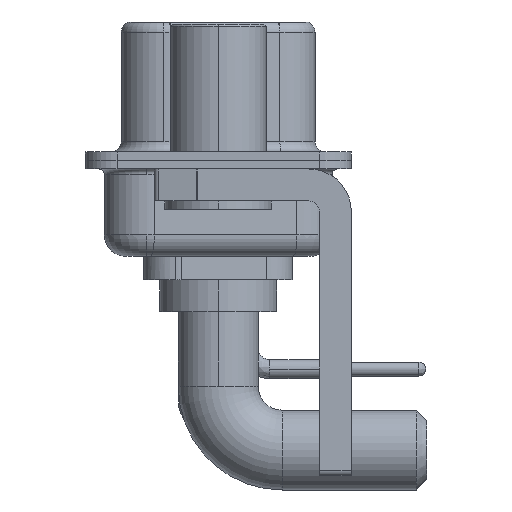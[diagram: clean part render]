
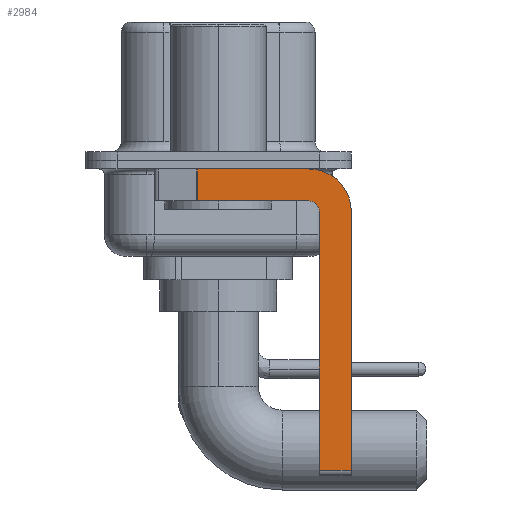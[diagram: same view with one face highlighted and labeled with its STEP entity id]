
A CAD part, left-side view. The second image highlights one B-rep face of the part: STEP entity #2984.
In plain terms, the highlighted planar face has unit normal (-1, 0, 0).
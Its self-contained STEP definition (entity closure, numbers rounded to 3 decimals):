
#46 = CARTESIAN_POINT ( 'NONE',  ( -2.9, -4.25, -2.4 ) ) ;
#227 = EDGE_CURVE ( 'NONE', #10229, #24073, #20370, .T. ) ;
#1025 = VERTEX_POINT ( 'NONE', #24218 ) ;
#1074 = CIRCLE ( 'NONE', #1941, 2. ) ;
#1205 = EDGE_CURVE ( 'NONE', #19453, #14094, #9927, .T. ) ;
#1941 = AXIS2_PLACEMENT_3D ( 'NONE', #13670, #17781, #24322 ) ;
#2048 = EDGE_CURVE ( 'NONE', #2101, #23943, #1074, .T. ) ;
#2101 = VERTEX_POINT ( 'NONE', #26499 ) ;
#2528 = LINE ( 'NONE', #2934, #19726 ) ;
#2921 = LINE ( 'NONE', #18061, #12128 ) ;
#2928 = CARTESIAN_POINT ( 'NONE',  ( -2.9, -4.75, -14.55 ) ) ;
#2934 = CARTESIAN_POINT ( 'NONE',  ( -2.9, -6.25, -2.4 ) ) ;
#2984 = ADVANCED_FACE ( 'NONE', ( #24904 ), #8509, .F. ) ;
#3278 = VERTEX_POINT ( 'NONE', #16267 ) ;
#3705 = DIRECTION ( 'NONE',  ( 0., 0., -1. ) ) ;
#4820 = DIRECTION ( 'NONE',  ( 0., -1., 0. ) ) ;
#5224 = DIRECTION ( 'NONE',  ( 0., 1., 0. ) ) ;
#5779 = EDGE_CURVE ( 'NONE', #1025, #3278, #6306, .T. ) ;
#5874 = AXIS2_PLACEMENT_3D ( 'NONE', #18556, #16498, #16630 ) ;
#6306 = CIRCLE ( 'NONE', #5874, 0.5 ) ;
#7132 = LINE ( 'NONE', #17126, #23671 ) ;
#7355 = EDGE_CURVE ( 'NONE', #19453, #1025, #18155, .T. ) ;
#7531 = ORIENTED_EDGE ( 'NONE', *, *, #17635, .F. ) ;
#7769 = CARTESIAN_POINT ( 'NONE',  ( -2.9, -4.75, -14.8 ) ) ;
#8048 = CARTESIAN_POINT ( 'NONE',  ( -2.9, 0.978, -0.4 ) ) ;
#8509 = PLANE ( 'NONE',  #12891 ) ;
#9927 = LINE ( 'NONE', #20561, #15841 ) ;
#10229 = VERTEX_POINT ( 'NONE', #8048 ) ;
#11127 = ORIENTED_EDGE ( 'NONE', *, *, #5779, .F. ) ;
#11384 = EDGE_CURVE ( 'NONE', #3278, #24073, #2921, .T. ) ;
#12128 = VECTOR ( 'NONE', #5224, 1000. ) ;
#12272 = ORIENTED_EDGE ( 'NONE', *, *, #1205, .T. ) ;
#12891 = AXIS2_PLACEMENT_3D ( 'NONE', #46, #14528, #22847 ) ;
#13019 = ORIENTED_EDGE ( 'NONE', *, *, #227, .T. ) ;
#13670 = CARTESIAN_POINT ( 'NONE',  ( -2.9, -4.25, -2.4 ) ) ;
#14094 = VERTEX_POINT ( 'NONE', #26295 ) ;
#14351 = CARTESIAN_POINT ( 'NONE',  ( -2.9, 0.978, -1.9 ) ) ;
#14528 = DIRECTION ( 'NONE',  ( 1., 0., 0. ) ) ;
#14727 = CARTESIAN_POINT ( 'NONE',  ( -2.9, 0.978, -1.9 ) ) ;
#15015 = VECTOR ( 'NONE', #16100, 1000. ) ;
#15141 = ORIENTED_EDGE ( 'NONE', *, *, #2048, .F. ) ;
#15361 = DIRECTION ( 'NONE',  ( 0., 0., -1. ) ) ;
#15841 = VECTOR ( 'NONE', #20299, 1000. ) ;
#16100 = DIRECTION ( 'NONE',  ( 0., 0., 1. ) ) ;
#16267 = CARTESIAN_POINT ( 'NONE',  ( -2.9, -4.25, -1.9 ) ) ;
#16498 = DIRECTION ( 'NONE',  ( -1., 0., 0. ) ) ;
#16630 = DIRECTION ( 'NONE',  ( 0., 0., 1. ) ) ;
#17126 = CARTESIAN_POINT ( 'NONE',  ( -2.9, 3., -0.4 ) ) ;
#17455 = EDGE_LOOP ( 'NONE', ( #7531, #13019, #19110, #11127, #19322, #12272, #23808, #15141 ) ) ;
#17635 = EDGE_CURVE ( 'NONE', #10229, #2101, #7132, .T. ) ;
#17781 = DIRECTION ( 'NONE',  ( 1., 0., 0. ) ) ;
#18061 = CARTESIAN_POINT ( 'NONE',  ( -2.9, -4.25, -1.9 ) ) ;
#18155 = LINE ( 'NONE', #7769, #15015 ) ;
#18556 = CARTESIAN_POINT ( 'NONE',  ( -2.9, -4.25, -2.4 ) ) ;
#19110 = ORIENTED_EDGE ( 'NONE', *, *, #11384, .F. ) ;
#19322 = ORIENTED_EDGE ( 'NONE', *, *, #7355, .F. ) ;
#19453 = VERTEX_POINT ( 'NONE', #2928 ) ;
#19726 = VECTOR ( 'NONE', #15361, 1000. ) ;
#20299 = DIRECTION ( 'NONE',  ( 0., -1., 0. ) ) ;
#20370 = LINE ( 'NONE', #14351, #24448 ) ;
#20561 = CARTESIAN_POINT ( 'NONE',  ( -2.9, -4.25, -14.55 ) ) ;
#20608 = CARTESIAN_POINT ( 'NONE',  ( -2.9, -6.25, -2.4 ) ) ;
#21354 = EDGE_CURVE ( 'NONE', #23943, #14094, #2528, .T. ) ;
#22847 = DIRECTION ( 'NONE',  ( 0., 0., -1. ) ) ;
#23671 = VECTOR ( 'NONE', #4820, 1000. ) ;
#23808 = ORIENTED_EDGE ( 'NONE', *, *, #21354, .F. ) ;
#23943 = VERTEX_POINT ( 'NONE', #20608 ) ;
#24073 = VERTEX_POINT ( 'NONE', #14727 ) ;
#24218 = CARTESIAN_POINT ( 'NONE',  ( -2.9, -4.75, -2.4 ) ) ;
#24322 = DIRECTION ( 'NONE',  ( 0., 0., -1. ) ) ;
#24448 = VECTOR ( 'NONE', #3705, 1000. ) ;
#24904 = FACE_OUTER_BOUND ( 'NONE', #17455, .T. ) ;
#26295 = CARTESIAN_POINT ( 'NONE',  ( -2.9, -6.25, -14.55 ) ) ;
#26499 = CARTESIAN_POINT ( 'NONE',  ( -2.9, -4.25, -0.4 ) ) ;
